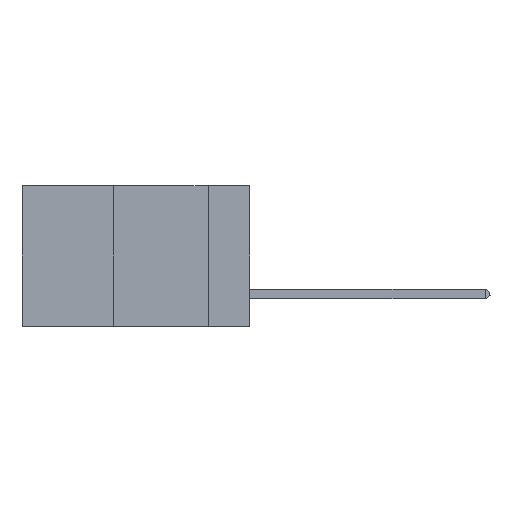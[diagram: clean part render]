
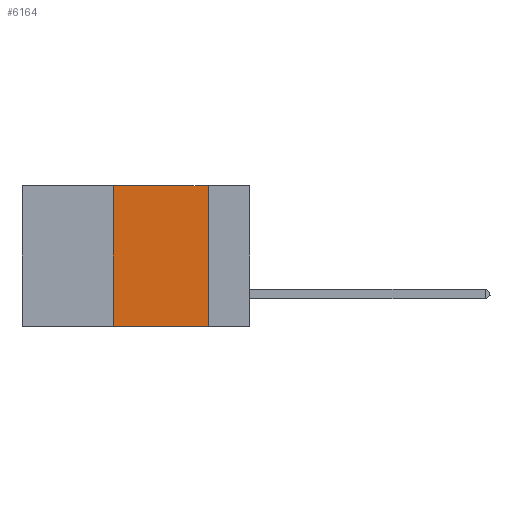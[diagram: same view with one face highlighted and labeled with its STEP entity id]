
A CAD part, left-side view. The second image highlights one B-rep face of the part: STEP entity #6164.
In plain terms, the highlighted planar face has unit normal (-1, 0, 0).
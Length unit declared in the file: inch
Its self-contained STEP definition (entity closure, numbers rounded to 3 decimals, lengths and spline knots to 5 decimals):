
#599 = CARTESIAN_POINT ( 'NONE',  ( 0., 0.36, 0. ) ) ;
#939 = PLANE ( 'NONE',  #1170 ) ;
#1058 = LINE ( 'NONE', #9945, #6526 ) ;
#1170 = AXIS2_PLACEMENT_3D ( 'NONE', #7717, #10731, #1913 ) ;
#1517 = CARTESIAN_POINT ( 'NONE',  ( 0., 0.36, 0. ) ) ;
#1913 = DIRECTION ( 'NONE',  ( 0., 0., -1. ) ) ;
#2608 = VERTEX_POINT ( 'NONE', #9495 ) ;
#2634 = VECTOR ( 'NONE', #8333, 39.37008 ) ;
#3018 = VERTEX_POINT ( 'NONE', #3800 ) ;
#3550 = CARTESIAN_POINT ( 'NONE',  ( 0., 0.11, -0.37 ) ) ;
#3800 = CARTESIAN_POINT ( 'NONE',  ( 0., 0.11, 0. ) ) ;
#3882 = CARTESIAN_POINT ( 'NONE',  ( 0., 0.6, -0.37 ) ) ;
#4188 = ORIENTED_EDGE ( 'NONE', *, *, #8824, .F. ) ;
#5298 = EDGE_CURVE ( 'NONE', #3018, #12063, #10202, .T. ) ;
#5572 = DIRECTION ( 'NONE',  ( 0., -1., 0. ) ) ;
#6164 = ADVANCED_FACE ( 'NONE', ( #11688 ), #939, .F. ) ;
#6470 = ORIENTED_EDGE ( 'NONE', *, *, #5298, .F. ) ;
#6526 = VECTOR ( 'NONE', #10918, 39.37008 ) ;
#6879 = EDGE_CURVE ( 'NONE', #11187, #3018, #1058, .T. ) ;
#7383 = DIRECTION ( 'NONE',  ( 0., 0., 1. ) ) ;
#7717 = CARTESIAN_POINT ( 'NONE',  ( 0., 0.6, 0. ) ) ;
#7804 = EDGE_LOOP ( 'NONE', ( #6470, #10665, #4188, #10952 ) ) ;
#8333 = DIRECTION ( 'NONE',  ( 0., 0., -1. ) ) ;
#8670 = VECTOR ( 'NONE', #5572, 39.37008 ) ;
#8824 = EDGE_CURVE ( 'NONE', #2608, #11187, #9893, .T. ) ;
#9449 = EDGE_CURVE ( 'NONE', #2608, #12063, #9730, .T. ) ;
#9495 = CARTESIAN_POINT ( 'NONE',  ( 0., 0.36, -0.37 ) ) ;
#9730 = LINE ( 'NONE', #3882, #8670 ) ;
#9893 = LINE ( 'NONE', #599, #10813 ) ;
#9945 = CARTESIAN_POINT ( 'NONE',  ( 0., 0.6, 0. ) ) ;
#10202 = LINE ( 'NONE', #10320, #2634 ) ;
#10320 = CARTESIAN_POINT ( 'NONE',  ( 0., 0.11, 0. ) ) ;
#10665 = ORIENTED_EDGE ( 'NONE', *, *, #6879, .F. ) ;
#10731 = DIRECTION ( 'NONE',  ( 1., 0., 0. ) ) ;
#10813 = VECTOR ( 'NONE', #7383, 39.37008 ) ;
#10918 = DIRECTION ( 'NONE',  ( 0., -1., 0. ) ) ;
#10952 = ORIENTED_EDGE ( 'NONE', *, *, #9449, .T. ) ;
#11187 = VERTEX_POINT ( 'NONE', #1517 ) ;
#11688 = FACE_OUTER_BOUND ( 'NONE', #7804, .T. ) ;
#12063 = VERTEX_POINT ( 'NONE', #3550 ) ;
